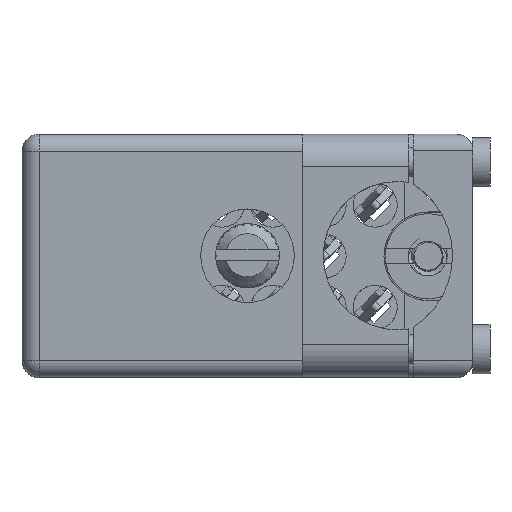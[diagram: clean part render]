
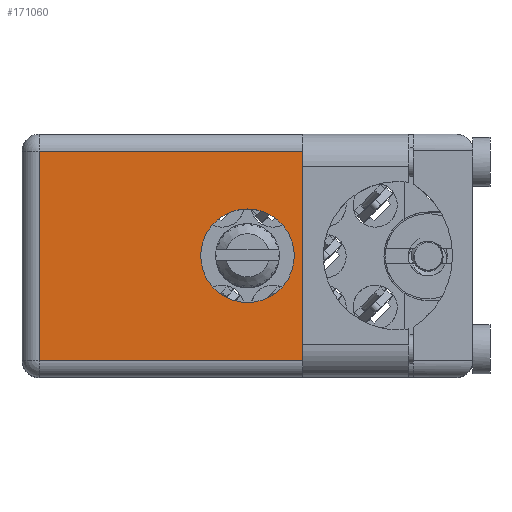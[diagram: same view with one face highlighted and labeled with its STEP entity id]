
A CAD part, top view. The second image highlights one B-rep face of the part: STEP entity #171060.
In plain terms, the highlighted face is planar.
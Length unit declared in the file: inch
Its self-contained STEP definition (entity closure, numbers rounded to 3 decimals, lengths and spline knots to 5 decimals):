
#1158 = CARTESIAN_POINT ( 'NONE',  ( 0.6625, 0.906, -0.3575 ) ) ;
#1798 = DIRECTION ( 'NONE',  ( 0., 1., 0. ) ) ;
#6525 = LINE ( 'NONE', #42103, #154939 ) ;
#7464 = EDGE_CURVE ( 'NONE', #191407, #9588, #171104, .T. ) ;
#9588 = VERTEX_POINT ( 'NONE', #135850 ) ;
#15516 = VECTOR ( 'NONE', #114358, 39.37008 ) ;
#19883 = VERTEX_POINT ( 'NONE', #50640 ) ;
#20635 = CARTESIAN_POINT ( 'NONE',  ( 1.15, 0.906, -0.05 ) ) ;
#21437 = VERTEX_POINT ( 'NONE', #114073 ) ;
#21874 = DIRECTION ( 'NONE',  ( 0., 1., 0. ) ) ;
#22024 = ORIENTED_EDGE ( 'NONE', *, *, #189329, .F. ) ;
#27913 = ORIENTED_EDGE ( 'NONE', *, *, #159477, .T. ) ;
#30434 = ORIENTED_EDGE ( 'NONE', *, *, #69103, .F. ) ;
#33123 = CARTESIAN_POINT ( 'NONE',  ( 1.15, 0.906, -0.715 ) ) ;
#38998 = CARTESIAN_POINT ( 'NONE',  ( 1.15, 0.906, -0.1125 ) ) ;
#39842 = LINE ( 'NONE', #146070, #84641 ) ;
#40620 = DIRECTION ( 'NONE',  ( 0., 0., -1. ) ) ;
#42103 = CARTESIAN_POINT ( 'NONE',  ( 0.865, 0.906, -0.1125 ) ) ;
#50640 = CARTESIAN_POINT ( 'NONE',  ( 0.05, 0.906, -0.665 ) ) ;
#52135 = CARTESIAN_POINT ( 'NONE',  ( 1.15, 0.906, -0.665 ) ) ;
#54984 = AXIS2_PLACEMENT_3D ( 'NONE', #1158, #1798, #106554 ) ;
#55658 = LINE ( 'NONE', #33123, #157010 ) ;
#56704 = VECTOR ( 'NONE', #186636, 39.37008 ) ;
#65363 = EDGE_LOOP ( 'NONE', ( #22024, #140569 ) ) ;
#69103 = EDGE_CURVE ( 'NONE', #71883, #152314, #55658, .T. ) ;
#71883 = VERTEX_POINT ( 'NONE', #52135 ) ;
#72284 = ORIENTED_EDGE ( 'NONE', *, *, #84945, .T. ) ;
#73333 = AXIS2_PLACEMENT_3D ( 'NONE', #87789, #101640, #162944 ) ;
#74483 = VERTEX_POINT ( 'NONE', #96213 ) ;
#77391 = EDGE_CURVE ( 'NONE', #71883, #19883, #91799, .T. ) ;
#78918 = ORIENTED_EDGE ( 'NONE', *, *, #128145, .T. ) ;
#80594 = ORIENTED_EDGE ( 'NONE', *, *, #7464, .F. ) ;
#83249 = FACE_BOUND ( 'NONE', #65363, .T. ) ;
#84641 = VECTOR ( 'NONE', #40620, 39.37008 ) ;
#84945 = EDGE_CURVE ( 'NONE', #74483, #9588, #113286, .T. ) ;
#87789 = CARTESIAN_POINT ( 'NONE',  ( 0.6625, 0.906, -0.3575 ) ) ;
#91799 = LINE ( 'NONE', #93513, #172004 ) ;
#92190 = VECTOR ( 'NONE', #109667, 39.37008 ) ;
#92685 = EDGE_CURVE ( 'NONE', #159760, #21437, #131779, .T. ) ;
#93128 = CARTESIAN_POINT ( 'NONE',  ( 0.05, 0.906, -0.715 ) ) ;
#93513 = CARTESIAN_POINT ( 'NONE',  ( 0., 0.906, -0.665 ) ) ;
#94178 = DIRECTION ( 'NONE',  ( -1., 0., 0. ) ) ;
#96213 = CARTESIAN_POINT ( 'NONE',  ( 0.05, 0.906, -0.05 ) ) ;
#98293 = CARTESIAN_POINT ( 'NONE',  ( 0., 0.906, -0.715 ) ) ;
#99182 = CARTESIAN_POINT ( 'NONE',  ( 1.15, 0.906, -0.715 ) ) ;
#101418 = EDGE_CURVE ( 'NONE', #19883, #74483, #193535, .T. ) ;
#101640 = DIRECTION ( 'NONE',  ( 0., 1., 0. ) ) ;
#105037 = CARTESIAN_POINT ( 'NONE',  ( 0.865, 0.906, -0.6025 ) ) ;
#106554 = DIRECTION ( 'NONE',  ( 0., 0., 1. ) ) ;
#109667 = DIRECTION ( 'NONE',  ( 0., 0., 1. ) ) ;
#112858 = DIRECTION ( 'NONE',  ( 0., 0., 1. ) ) ;
#113286 = LINE ( 'NONE', #20635, #56704 ) ;
#114073 = CARTESIAN_POINT ( 'NONE',  ( 0.6625, 0.906, -0.22 ) ) ;
#114358 = DIRECTION ( 'NONE',  ( 0., 0., 1. ) ) ;
#115372 = CARTESIAN_POINT ( 'NONE',  ( 0.865, 0.906, -0.1125 ) ) ;
#115523 = CARTESIAN_POINT ( 'NONE',  ( 0.865, 0.906, -0.6025 ) ) ;
#120293 = VECTOR ( 'NONE', #133262, 39.37008 ) ;
#128145 = EDGE_CURVE ( 'NONE', #162173, #164185, #39842, .T. ) ;
#129235 = DIRECTION ( 'NONE',  ( 0., 0., 1. ) ) ;
#131779 = CIRCLE ( 'NONE', #73333, 0.1375 ) ;
#133262 = DIRECTION ( 'NONE',  ( 1., 0., 0. ) ) ;
#135850 = CARTESIAN_POINT ( 'NONE',  ( 1.15, 0.906, -0.05 ) ) ;
#137672 = ORIENTED_EDGE ( 'NONE', *, *, #155173, .T. ) ;
#139783 = FACE_OUTER_BOUND ( 'NONE', #181381, .T. ) ;
#140569 = ORIENTED_EDGE ( 'NONE', *, *, #92685, .F. ) ;
#142491 = PLANE ( 'NONE',  #193242 ) ;
#146070 = CARTESIAN_POINT ( 'NONE',  ( 0.865, 0.906, -0.1125 ) ) ;
#148181 = CARTESIAN_POINT ( 'NONE',  ( 0.6625, 0.906, -0.495 ) ) ;
#148205 = DIRECTION ( 'NONE',  ( -1., 0., 0. ) ) ;
#152314 = VERTEX_POINT ( 'NONE', #158346 ) ;
#154939 = VECTOR ( 'NONE', #148205, 39.37008 ) ;
#155173 = EDGE_CURVE ( 'NONE', #191407, #162173, #6525, .T. ) ;
#157010 = VECTOR ( 'NONE', #112858, 39.37008 ) ;
#158113 = CIRCLE ( 'NONE', #54984, 0.1375 ) ;
#158346 = CARTESIAN_POINT ( 'NONE',  ( 1.15, 0.906, -0.6025 ) ) ;
#159477 = EDGE_CURVE ( 'NONE', #164185, #152314, #160411, .T. ) ;
#159760 = VERTEX_POINT ( 'NONE', #148181 ) ;
#160411 = LINE ( 'NONE', #115523, #120293 ) ;
#161643 = ORIENTED_EDGE ( 'NONE', *, *, #101418, .T. ) ;
#162173 = VERTEX_POINT ( 'NONE', #115372 ) ;
#162944 = DIRECTION ( 'NONE',  ( 0., 0., 1. ) ) ;
#164185 = VERTEX_POINT ( 'NONE', #105037 ) ;
#168584 = ORIENTED_EDGE ( 'NONE', *, *, #77391, .T. ) ;
#171060 = ADVANCED_FACE ( 'NONE', ( #139783, #83249 ), #142491, .T. ) ;
#171104 = LINE ( 'NONE', #99182, #15516 ) ;
#172004 = VECTOR ( 'NONE', #94178, 39.37008 ) ;
#181381 = EDGE_LOOP ( 'NONE', ( #161643, #72284, #80594, #137672, #78918, #27913, #30434, #168584 ) ) ;
#186636 = DIRECTION ( 'NONE',  ( 1., 0., 0. ) ) ;
#189329 = EDGE_CURVE ( 'NONE', #21437, #159760, #158113, .T. ) ;
#191407 = VERTEX_POINT ( 'NONE', #38998 ) ;
#193242 = AXIS2_PLACEMENT_3D ( 'NONE', #98293, #21874, #129235 ) ;
#193535 = LINE ( 'NONE', #93128, #92190 ) ;
